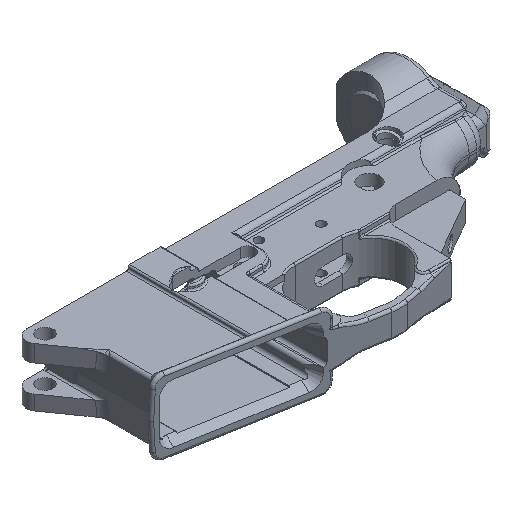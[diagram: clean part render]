
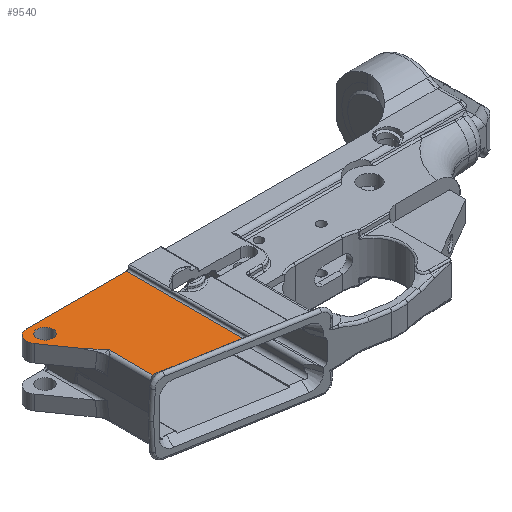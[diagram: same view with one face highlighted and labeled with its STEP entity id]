
A CAD part, isometric view. The second image highlights one B-rep face of the part: STEP entity #9540.
In plain terms, the highlighted planar face has unit normal (0, 0, 1).
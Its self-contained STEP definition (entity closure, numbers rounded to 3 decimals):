
#185=FACE_BOUND('',#1968,.T.);
#366=B_SPLINE_CURVE_WITH_KNOTS('',3,(#17102,#17103,#17104,#17105,#17106,
#17107),.UNSPECIFIED.,.F.,.F.,(4,2,4),(-0.114,-0.051,
0.),.UNSPECIFIED.);
#458=B_SPLINE_CURVE_WITH_KNOTS('',3,(#21962,#21963,#21964,#21965,#21966,
#21967,#21968,#21969,#21970,#21971,#21972,#21973,#21974,#21975),
 .UNSPECIFIED.,.F.,.F.,(4,2,2,2,2,2,4),(-0.993,-0.797,
-0.381,-0.24,-0.093,0.,0.017),
 .UNSPECIFIED.);
#881=PLANE('',#10498);
#1400=FACE_OUTER_BOUND('',#1967,.T.);
#1967=EDGE_LOOP('',(#8865,#8866,#8867,#8868,#8869,#8870,#8871,#8872));
#1968=EDGE_LOOP('',(#8873));
#2278=LINE('',#15555,#2985);
#2388=LINE('',#16589,#3095);
#2546=LINE('',#18645,#3253);
#2673=LINE('',#21604,#3380);
#2690=LINE('',#22073,#3397);
#2985=VECTOR('',#11541,35.853);
#3095=VECTOR('',#11877,54.9);
#3253=VECTOR('',#12463,20.718);
#3380=VECTOR('',#13022,10.);
#3397=VECTOR('',#13087,37.251);
#3710=CIRCLE('',#10262,3.738);
#3810=CIRCLE('',#10499,5.);
#4211=VERTEX_POINT('',#15552);
#4212=VERTEX_POINT('',#15554);
#4353=VERTEX_POINT('',#16587);
#4449=VERTEX_POINT('',#17101);
#4532=VERTEX_POINT('',#18511);
#4537=VERTEX_POINT('',#18649);
#4706=VERTEX_POINT('',#21594);
#4707=VERTEX_POINT('',#21597);
#4720=VERTEX_POINT('',#22071);
#5283=EDGE_CURVE('',#4211,#4212,#2278,.T.);
#5485=EDGE_CURVE('',#4353,#4211,#2388,.T.);
#5640=EDGE_CURVE('',#4212,#4449,#366,.T.);
#5798=EDGE_CURVE('',#4449,#4532,#2546,.T.);
#5801=EDGE_CURVE('',#4537,#4537,#3710,.T.);
#6106=EDGE_CURVE('',#4707,#4706,#2673,.T.);
#6107=EDGE_CURVE('',#4707,#4532,#458,.T.);
#6136=EDGE_CURVE('',#4706,#4720,#3810,.T.);
#6137=EDGE_CURVE('',#4720,#4353,#2690,.T.);
#8865=ORIENTED_EDGE('',*,*,#6136,.F.);
#8866=ORIENTED_EDGE('',*,*,#6106,.F.);
#8867=ORIENTED_EDGE('',*,*,#6107,.T.);
#8868=ORIENTED_EDGE('',*,*,#5798,.F.);
#8869=ORIENTED_EDGE('',*,*,#5640,.F.);
#8870=ORIENTED_EDGE('',*,*,#5283,.F.);
#8871=ORIENTED_EDGE('',*,*,#5485,.F.);
#8872=ORIENTED_EDGE('',*,*,#6137,.F.);
#8873=ORIENTED_EDGE('',*,*,#5801,.T.);
#9540=ADVANCED_FACE('',(#1400,#185),#881,.F.);
#10262=AXIS2_PLACEMENT_3D('',#18651,#12469,#12470);
#10498=AXIS2_PLACEMENT_3D('',#22070,#13083,#13084);
#10499=AXIS2_PLACEMENT_3D('',#22072,#13085,#13086);
#11541=DIRECTION('',(-0.985,0.174,0.));
#11877=DIRECTION('',(0.,-1.,0.));
#12463=DIRECTION('',(0.,1.,0.));
#12469=DIRECTION('center_axis',(0.,0.,
-1.));
#12470=DIRECTION('ref_axis',(0.,-1.,0.));
#13022=DIRECTION('',(-0.574,0.819,0.));
#13083=DIRECTION('center_axis',(0.,0.,
-1.));
#13084=DIRECTION('ref_axis',(0.,-1.,0.));
#13085=DIRECTION('center_axis',(0.,0.,
-1.));
#13086=DIRECTION('ref_axis',(0.,1.,0.));
#13087=DIRECTION('',(1.,0.,0.));
#15552=CARTESIAN_POINT('',(444.425,113.133,28.017));
#15554=CARTESIAN_POINT('',(409.116,119.359,28.017));
#15555=CARTESIAN_POINT('',(444.425,113.133,28.017));
#16587=CARTESIAN_POINT('',(444.425,168.033,28.017));
#16589=CARTESIAN_POINT('',(444.425,168.033,28.017));
#17101=CARTESIAN_POINT('',(408.113,119.207,28.017));
#17102=CARTESIAN_POINT('Ctrl Pts',(409.116,119.359,28.017));
#17103=CARTESIAN_POINT('Ctrl Pts',(408.978,119.383,28.017));
#17104=CARTESIAN_POINT('Ctrl Pts',(408.811,119.39,28.017));
#17105=CARTESIAN_POINT('Ctrl Pts',(408.437,119.324,28.017));
#17106=CARTESIAN_POINT('Ctrl Pts',(408.271,119.271,28.017));
#17107=CARTESIAN_POINT('Ctrl Pts',(408.113,119.207,28.017));
#18511=CARTESIAN_POINT('',(408.113,139.925,28.017));
#18645=CARTESIAN_POINT('',(408.113,119.207,28.017));
#18649=CARTESIAN_POINT('',(399.594,165.421,28.017));
#18651=CARTESIAN_POINT('Origin',(399.594,161.683,28.017));
#21594=CARTESIAN_POINT('',(393.011,160.165,28.017));
#21597=CARTESIAN_POINT('',(402.245,146.977,28.017));
#21604=CARTESIAN_POINT('',(412.142,132.844,28.017));
#21962=CARTESIAN_POINT('Ctrl Pts',(402.245,146.977,28.017));
#21963=CARTESIAN_POINT('Ctrl Pts',(402.546,146.596,28.017));
#21964=CARTESIAN_POINT('Ctrl Pts',(402.834,146.235,28.017));
#21965=CARTESIAN_POINT('Ctrl Pts',(403.955,144.841,28.017));
#21966=CARTESIAN_POINT('Ctrl Pts',(404.497,144.185,28.017));
#21967=CARTESIAN_POINT('Ctrl Pts',(405.715,142.754,28.017));
#21968=CARTESIAN_POINT('Ctrl Pts',(406.035,142.38,28.017));
#21969=CARTESIAN_POINT('Ctrl Pts',(406.741,141.551,28.017));
#21970=CARTESIAN_POINT('Ctrl Pts',(407.044,141.193,28.017));
#21971=CARTESIAN_POINT('Ctrl Pts',(407.591,140.545,28.017));
#21972=CARTESIAN_POINT('Ctrl Pts',(407.804,140.293,28.017));
#21973=CARTESIAN_POINT('Ctrl Pts',(408.041,140.012,28.017));
#21974=CARTESIAN_POINT('Ctrl Pts',(408.077,139.969,28.017));
#21975=CARTESIAN_POINT('Ctrl Pts',(408.113,139.925,28.017));
#22070=CARTESIAN_POINT('Origin',(419.723,112.804,28.017));
#22071=CARTESIAN_POINT('',(397.107,168.033,28.017));
#22072=CARTESIAN_POINT('Origin',(397.107,163.033,28.017));
#22073=CARTESIAN_POINT('',(407.173,168.033,28.017));
